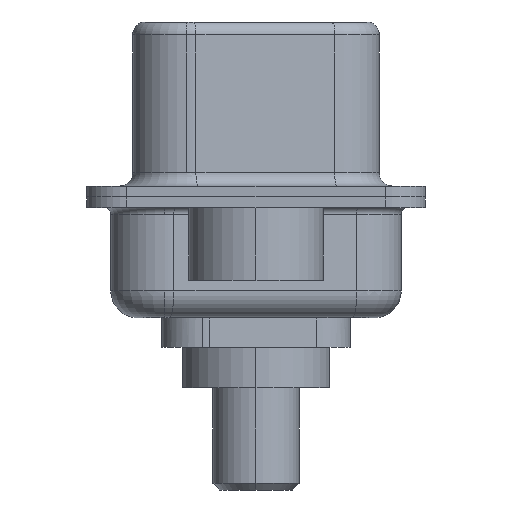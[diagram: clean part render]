
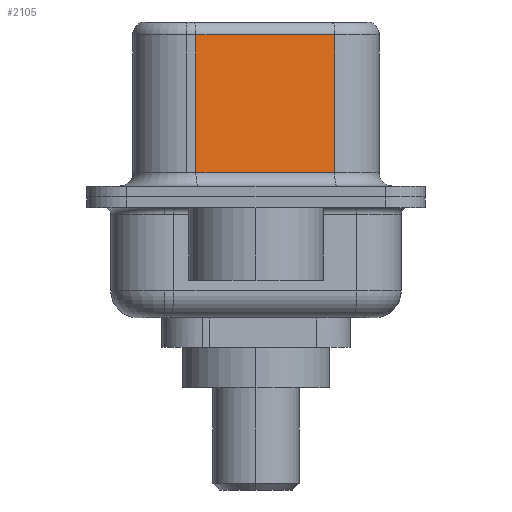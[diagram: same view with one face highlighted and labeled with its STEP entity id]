
A CAD part, left-side view. The second image highlights one B-rep face of the part: STEP entity #2105.
In plain terms, the highlighted planar face has unit normal (-0.985, -0.174, 0).
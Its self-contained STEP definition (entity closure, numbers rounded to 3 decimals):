
#228 = DIRECTION ( 'NONE',  ( 0., 0., -1. ) ) ;
#425 = CARTESIAN_POINT ( 'NONE',  ( 4.585, -2.927, 6.52 ) ) ;
#1821 = EDGE_CURVE ( 'NONE', #11876, #7876, #9498, .T. ) ;
#2105 = ADVANCED_FACE ( 'NONE', ( #17059 ), #13899, .F. ) ;
#2369 = EDGE_LOOP ( 'NONE', ( #14424, #13374, #4665, #11161 ) ) ;
#2721 = CARTESIAN_POINT ( 'NONE',  ( 4.585, -2.927, 0.9 ) ) ;
#4665 = ORIENTED_EDGE ( 'NONE', *, *, #1821, .T. ) ;
#4735 = CARTESIAN_POINT ( 'NONE',  ( 3.675, 2.233, 0.9 ) ) ;
#5427 = DIRECTION ( 'NONE',  ( 0.985, 0.174, 0. ) ) ;
#6544 = VECTOR ( 'NONE', #228, 1000. ) ;
#6727 = DIRECTION ( 'NONE',  ( 0.174, -0.985, 0. ) ) ;
#7650 = LINE ( 'NONE', #16244, #10638 ) ;
#7811 = LINE ( 'NONE', #2721, #15069 ) ;
#7876 = VERTEX_POINT ( 'NONE', #4735 ) ;
#8019 = AXIS2_PLACEMENT_3D ( 'NONE', #8451, #5427, #11199 ) ;
#8357 = VERTEX_POINT ( 'NONE', #10122 ) ;
#8450 = DIRECTION ( 'NONE',  ( -0.174, 0.985, 0. ) ) ;
#8451 = CARTESIAN_POINT ( 'NONE',  ( 4.585, -2.927, 6.52 ) ) ;
#8947 = VECTOR ( 'NONE', #13578, 1000. ) ;
#9165 = EDGE_CURVE ( 'NONE', #7876, #8357, #7811, .T. ) ;
#9498 = LINE ( 'NONE', #11711, #6544 ) ;
#10122 = CARTESIAN_POINT ( 'NONE',  ( 4.585, -2.927, 0.9 ) ) ;
#10638 = VECTOR ( 'NONE', #8450, 1000. ) ;
#11161 = ORIENTED_EDGE ( 'NONE', *, *, #9165, .T. ) ;
#11199 = DIRECTION ( 'NONE',  ( -0.174, 0.985, 0. ) ) ;
#11711 = CARTESIAN_POINT ( 'NONE',  ( 3.675, 2.233, 6.52 ) ) ;
#11768 = EDGE_CURVE ( 'NONE', #16720, #8357, #15879, .T. ) ;
#11876 = VERTEX_POINT ( 'NONE', #15036 ) ;
#13374 = ORIENTED_EDGE ( 'NONE', *, *, #16036, .T. ) ;
#13578 = DIRECTION ( 'NONE',  ( 0., 0., -1. ) ) ;
#13899 = PLANE ( 'NONE',  #8019 ) ;
#14424 = ORIENTED_EDGE ( 'NONE', *, *, #11768, .F. ) ;
#15036 = CARTESIAN_POINT ( 'NONE',  ( 3.675, 2.233, 6.02 ) ) ;
#15069 = VECTOR ( 'NONE', #6727, 1000. ) ;
#15153 = CARTESIAN_POINT ( 'NONE',  ( 4.585, -2.927, 6.02 ) ) ;
#15879 = LINE ( 'NONE', #425, #8947 ) ;
#16036 = EDGE_CURVE ( 'NONE', #16720, #11876, #7650, .T. ) ;
#16244 = CARTESIAN_POINT ( 'NONE',  ( 4.585, -2.927, 6.02 ) ) ;
#16720 = VERTEX_POINT ( 'NONE', #15153 ) ;
#17059 = FACE_OUTER_BOUND ( 'NONE', #2369, .T. ) ;
